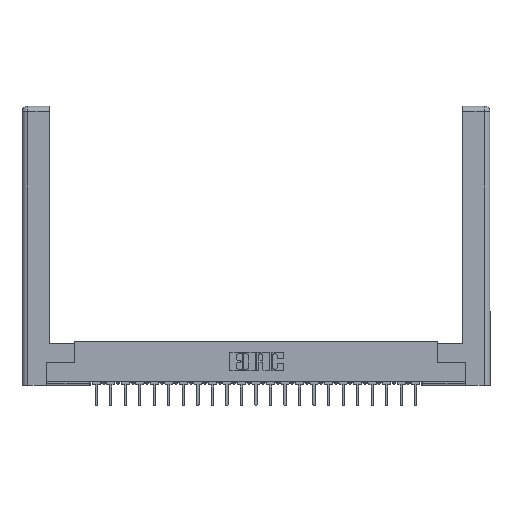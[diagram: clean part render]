
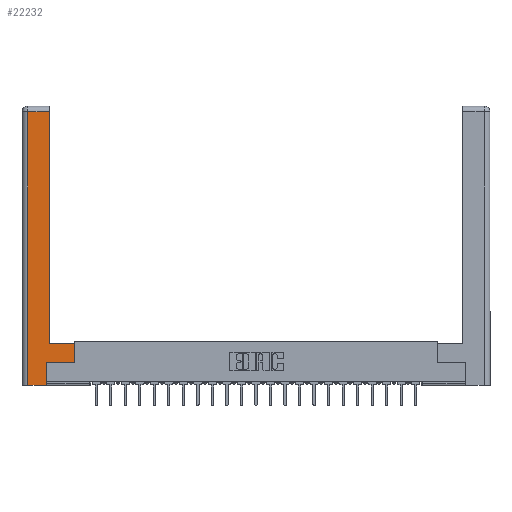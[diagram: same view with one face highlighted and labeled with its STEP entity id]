
A CAD part, top view. The second image highlights one B-rep face of the part: STEP entity #22232.
In plain terms, the highlighted planar face has unit normal (0, 0, 1).
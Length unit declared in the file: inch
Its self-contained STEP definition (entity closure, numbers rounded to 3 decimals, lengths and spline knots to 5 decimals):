
#120 = DIRECTION ( 'NONE',  ( 0., 1., 0. ) ) ;
#354 = EDGE_CURVE ( 'NONE', #8227, #5769, #19007, .T. ) ;
#359 = ORIENTED_EDGE ( 'NONE', *, *, #2296, .T. ) ;
#713 = ORIENTED_EDGE ( 'NONE', *, *, #11074, .T. ) ;
#1066 = VECTOR ( 'NONE', #7406, 39.37008 ) ;
#1446 = EDGE_CURVE ( 'NONE', #2369, #22407, #1769, .T. ) ;
#1769 = LINE ( 'NONE', #4271, #21094 ) ;
#1850 = CARTESIAN_POINT ( 'NONE',  ( 0.565, 0.245, 0. ) ) ;
#2296 = EDGE_CURVE ( 'NONE', #8123, #14544, #5421, .T. ) ;
#2366 = DIRECTION ( 'NONE',  ( 0., 1., 0. ) ) ;
#2369 = VERTEX_POINT ( 'NONE', #18862 ) ;
#3439 = DIRECTION ( 'NONE',  ( -1., 0., 0. ) ) ;
#4253 = CARTESIAN_POINT ( 'NONE',  ( 0.295, 3., 0. ) ) ;
#4271 = CARTESIAN_POINT ( 'NONE',  ( 0.0615, 0., 0. ) ) ;
#5144 = VECTOR ( 'NONE', #16142, 39.37008 ) ;
#5383 = EDGE_CURVE ( 'NONE', #5769, #9998, #18759, .T. ) ;
#5421 = LINE ( 'NONE', #6654, #23501 ) ;
#5769 = VERTEX_POINT ( 'NONE', #8690 ) ;
#5914 = ORIENTED_EDGE ( 'NONE', *, *, #1446, .T. ) ;
#5966 = VERTEX_POINT ( 'NONE', #7141 ) ;
#6118 = AXIS2_PLACEMENT_3D ( 'NONE', #17543, #21203, #15595 ) ;
#6654 = CARTESIAN_POINT ( 'NONE',  ( 0.265, 0.245, 0. ) ) ;
#6660 = CARTESIAN_POINT ( 'NONE',  ( 0.295, 0.45, 0. ) ) ;
#7141 = CARTESIAN_POINT ( 'NONE',  ( 0.295, 2.94, 0. ) ) ;
#7406 = DIRECTION ( 'NONE',  ( -1., 0., 0. ) ) ;
#7573 = ORIENTED_EDGE ( 'NONE', *, *, #354, .T. ) ;
#8078 = CARTESIAN_POINT ( 'NONE',  ( 0.0615, 0., 0. ) ) ;
#8123 = VERTEX_POINT ( 'NONE', #24128 ) ;
#8227 = VERTEX_POINT ( 'NONE', #1850 ) ;
#8228 = FACE_OUTER_BOUND ( 'NONE', #16631, .T. ) ;
#8640 = VECTOR ( 'NONE', #120, 39.37008 ) ;
#8690 = CARTESIAN_POINT ( 'NONE',  ( 0.565, 0.45, 0. ) ) ;
#9163 = EDGE_CURVE ( 'NONE', #5966, #2369, #17355, .T. ) ;
#9530 = PLANE ( 'NONE',  #6118 ) ;
#9535 = CARTESIAN_POINT ( 'NONE',  ( 0.0615, 2.94, 0. ) ) ;
#9998 = VERTEX_POINT ( 'NONE', #6660 ) ;
#10626 = ORIENTED_EDGE ( 'NONE', *, *, #25168, .T. ) ;
#10651 = VECTOR ( 'NONE', #20147, 39.37008 ) ;
#11008 = LINE ( 'NONE', #19939, #5144 ) ;
#11074 = EDGE_CURVE ( 'NONE', #22407, #8123, #11008, .T. ) ;
#11388 = ORIENTED_EDGE ( 'NONE', *, *, #25309, .T. ) ;
#11822 = CARTESIAN_POINT ( 'NONE',  ( 0.265, 0.245, 0. ) ) ;
#12182 = LINE ( 'NONE', #24112, #10651 ) ;
#12205 = VECTOR ( 'NONE', #2366, 39.37008 ) ;
#14469 = DIRECTION ( 'NONE',  ( 0., 1., 0. ) ) ;
#14544 = VERTEX_POINT ( 'NONE', #11822 ) ;
#15595 = DIRECTION ( 'NONE',  ( -1., 0., 0. ) ) ;
#15790 = CARTESIAN_POINT ( 'NONE',  ( 0.565, 0.45, 0. ) ) ;
#16133 = DIRECTION ( 'NONE',  ( 0., -1., 0. ) ) ;
#16142 = DIRECTION ( 'NONE',  ( 1., 0., 0. ) ) ;
#16345 = VECTOR ( 'NONE', #3439, 39.37008 ) ;
#16631 = EDGE_LOOP ( 'NONE', ( #10626, #22820, #5914, #713, #359, #11388, #7573, #21630 ) ) ;
#17355 = LINE ( 'NONE', #9535, #1066 ) ;
#17373 = LINE ( 'NONE', #4253, #12205 ) ;
#17543 = CARTESIAN_POINT ( 'NONE',  ( 0., 0., 0. ) ) ;
#18759 = LINE ( 'NONE', #23056, #16345 ) ;
#18862 = CARTESIAN_POINT ( 'NONE',  ( 0.0615, 2.94, 0. ) ) ;
#19007 = LINE ( 'NONE', #15790, #8640 ) ;
#19939 = CARTESIAN_POINT ( 'NONE',  ( 0.265, 0., 0. ) ) ;
#20147 = DIRECTION ( 'NONE',  ( 1., 0., 0. ) ) ;
#21094 = VECTOR ( 'NONE', #16133, 39.37008 ) ;
#21203 = DIRECTION ( 'NONE',  ( 0., 0., -1. ) ) ;
#21630 = ORIENTED_EDGE ( 'NONE', *, *, #5383, .T. ) ;
#22232 = ADVANCED_FACE ( 'NONE', ( #8228 ), #9530, .F. ) ;
#22407 = VERTEX_POINT ( 'NONE', #8078 ) ;
#22820 = ORIENTED_EDGE ( 'NONE', *, *, #9163, .T. ) ;
#23056 = CARTESIAN_POINT ( 'NONE',  ( 0.295, 0.45, 0. ) ) ;
#23501 = VECTOR ( 'NONE', #14469, 39.37008 ) ;
#24112 = CARTESIAN_POINT ( 'NONE',  ( 0.565, 0.245, 0. ) ) ;
#24128 = CARTESIAN_POINT ( 'NONE',  ( 0.265, 0., 0. ) ) ;
#25168 = EDGE_CURVE ( 'NONE', #9998, #5966, #17373, .T. ) ;
#25309 = EDGE_CURVE ( 'NONE', #14544, #8227, #12182, .T. ) ;
